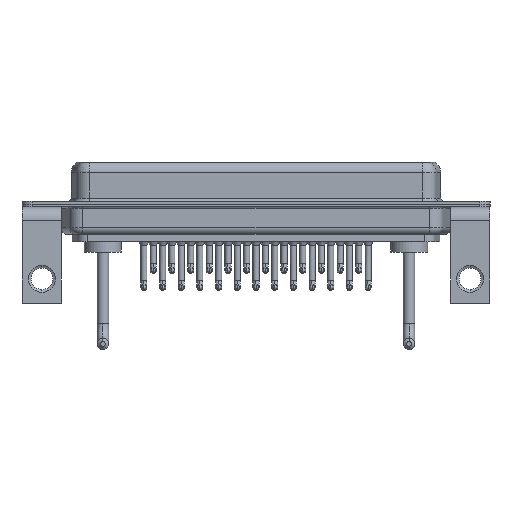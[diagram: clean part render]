
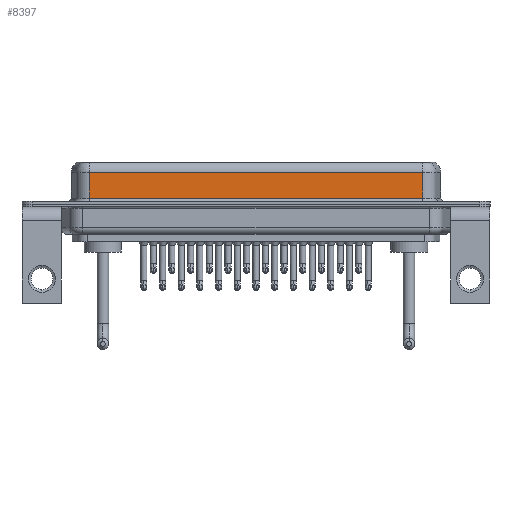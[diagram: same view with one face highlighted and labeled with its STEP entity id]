
A CAD part, front view. The second image highlights one B-rep face of the part: STEP entity #8397.
In plain terms, the highlighted planar face has unit normal (0, -1, 0).
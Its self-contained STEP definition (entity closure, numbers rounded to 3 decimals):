
#535 = CARTESIAN_POINT ( 'NONE',  ( 7.038, -3.95, 4.65 ) ) ;
#857 = EDGE_CURVE ( 'NONE', #24556, #25171, #18241, .T. ) ;
#2310 = VERTEX_POINT ( 'NONE', #23962 ) ;
#3321 = CARTESIAN_POINT ( 'NONE',  ( 56.462, -3.95, 0.9 ) ) ;
#4595 = DIRECTION ( 'NONE',  ( 0., 0., -1. ) ) ;
#4758 = DIRECTION ( 'NONE',  ( -1., 0., 0. ) ) ;
#5264 = DIRECTION ( 'NONE',  ( 1., 0., 0. ) ) ;
#5574 = FACE_OUTER_BOUND ( 'NONE', #7690, .T. ) ;
#5718 = AXIS2_PLACEMENT_3D ( 'NONE', #15687, #23581, #19712 ) ;
#6428 = CARTESIAN_POINT ( 'NONE',  ( 56.462, -3.95, 4.65 ) ) ;
#7400 = CARTESIAN_POINT ( 'NONE',  ( 7.038, -3.95, 6.4 ) ) ;
#7587 = LINE ( 'NONE', #3321, #17442 ) ;
#7661 = VERTEX_POINT ( 'NONE', #10564 ) ;
#7690 = EDGE_LOOP ( 'NONE', ( #10396, #17459, #13665, #21106 ) ) ;
#7978 = VECTOR ( 'NONE', #4595, 1000. ) ;
#8397 = ADVANCED_FACE ( 'NONE', ( #5574 ), #11684, .F. ) ;
#9236 = LINE ( 'NONE', #7400, #15143 ) ;
#10396 = ORIENTED_EDGE ( 'NONE', *, *, #22769, .F. ) ;
#10564 = CARTESIAN_POINT ( 'NONE',  ( 7.038, -3.95, 0.9 ) ) ;
#10704 = LINE ( 'NONE', #12903, #7978 ) ;
#10808 = CARTESIAN_POINT ( 'NONE',  ( 56.462, -3.95, 4.65 ) ) ;
#11684 = PLANE ( 'NONE',  #5718 ) ;
#12903 = CARTESIAN_POINT ( 'NONE',  ( 56.462, -3.95, 6.4 ) ) ;
#13665 = ORIENTED_EDGE ( 'NONE', *, *, #24884, .T. ) ;
#15143 = VECTOR ( 'NONE', #23218, 1000. ) ;
#15687 = CARTESIAN_POINT ( 'NONE',  ( 56.462, -3.95, 6.4 ) ) ;
#17442 = VECTOR ( 'NONE', #5264, 1000. ) ;
#17459 = ORIENTED_EDGE ( 'NONE', *, *, #857, .T. ) ;
#18241 = LINE ( 'NONE', #6428, #22993 ) ;
#19422 = EDGE_CURVE ( 'NONE', #7661, #2310, #7587, .T. ) ;
#19712 = DIRECTION ( 'NONE',  ( 0., 0., 1. ) ) ;
#21106 = ORIENTED_EDGE ( 'NONE', *, *, #19422, .T. ) ;
#22769 = EDGE_CURVE ( 'NONE', #24556, #2310, #10704, .T. ) ;
#22993 = VECTOR ( 'NONE', #4758, 1000. ) ;
#23218 = DIRECTION ( 'NONE',  ( 0., 0., -1. ) ) ;
#23581 = DIRECTION ( 'NONE',  ( 0., 1., 0. ) ) ;
#23962 = CARTESIAN_POINT ( 'NONE',  ( 56.462, -3.95, 0.9 ) ) ;
#24556 = VERTEX_POINT ( 'NONE', #10808 ) ;
#24884 = EDGE_CURVE ( 'NONE', #25171, #7661, #9236, .T. ) ;
#25171 = VERTEX_POINT ( 'NONE', #535 ) ;
